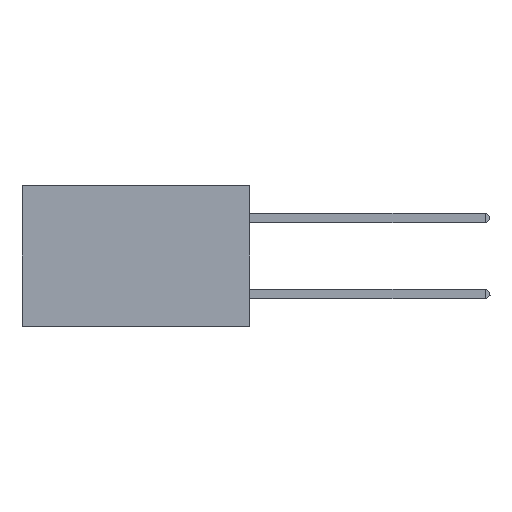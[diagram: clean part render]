
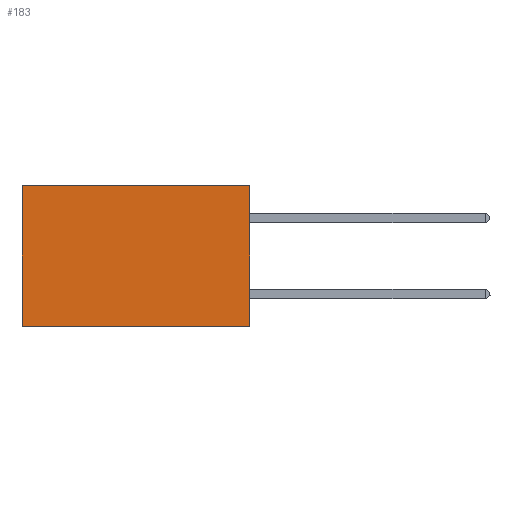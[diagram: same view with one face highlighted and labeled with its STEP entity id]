
A CAD part, left-side view. The second image highlights one B-rep face of the part: STEP entity #183.
In plain terms, the highlighted planar face has unit normal (-1, 0, 0).
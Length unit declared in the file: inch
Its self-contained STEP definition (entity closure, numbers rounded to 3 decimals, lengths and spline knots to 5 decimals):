
#183 = ADVANCED_FACE ( 'NONE', ( #19137 ), #21344, .F. ) ;
#465 = LINE ( 'NONE', #4104, #26621 ) ;
#587 = VECTOR ( 'NONE', #28675, 39.37008 ) ;
#904 = VERTEX_POINT ( 'NONE', #18651 ) ;
#2694 = AXIS2_PLACEMENT_3D ( 'NONE', #28165, #21142, #10325 ) ;
#4104 = CARTESIAN_POINT ( 'NONE',  ( 0.2875, 0.6, 0. ) ) ;
#4763 = ORIENTED_EDGE ( 'NONE', *, *, #7177, .T. ) ;
#5711 = DIRECTION ( 'NONE',  ( 0., 0., -1. ) ) ;
#6086 = VECTOR ( 'NONE', #22652, 39.37008 ) ;
#6959 = VECTOR ( 'NONE', #5711, 39.37008 ) ;
#7177 = EDGE_CURVE ( 'NONE', #10884, #16559, #465, .T. ) ;
#7529 = LINE ( 'NONE', #8794, #587 ) ;
#7625 = CARTESIAN_POINT ( 'NONE',  ( 0.2875, 0.6, 0. ) ) ;
#7751 = DIRECTION ( 'NONE',  ( 0., 0., -1. ) ) ;
#8175 = CARTESIAN_POINT ( 'NONE',  ( 0.2875, 0.6, -0.37 ) ) ;
#8794 = CARTESIAN_POINT ( 'NONE',  ( 0.2875, 0., -0.37 ) ) ;
#9261 = EDGE_CURVE ( 'NONE', #904, #20827, #15377, .T. ) ;
#9324 = EDGE_LOOP ( 'NONE', ( #4763, #24900, #26496, #24456 ) ) ;
#9924 = CARTESIAN_POINT ( 'NONE',  ( 0.2875, 0., 0. ) ) ;
#10039 = CARTESIAN_POINT ( 'NONE',  ( 0.2875, 0., -0.37 ) ) ;
#10325 = DIRECTION ( 'NONE',  ( 0., 0., -1. ) ) ;
#10884 = VERTEX_POINT ( 'NONE', #7625 ) ;
#14539 = EDGE_CURVE ( 'NONE', #904, #10884, #24881, .T. ) ;
#15377 = LINE ( 'NONE', #27958, #6959 ) ;
#16559 = VERTEX_POINT ( 'NONE', #8175 ) ;
#18651 = CARTESIAN_POINT ( 'NONE',  ( 0.2875, 0., 0. ) ) ;
#19137 = FACE_OUTER_BOUND ( 'NONE', #9324, .T. ) ;
#20827 = VERTEX_POINT ( 'NONE', #10039 ) ;
#21142 = DIRECTION ( 'NONE',  ( 1., 0., 0. ) ) ;
#21344 = PLANE ( 'NONE',  #2694 ) ;
#22652 = DIRECTION ( 'NONE',  ( 0., 1., 0. ) ) ;
#24456 = ORIENTED_EDGE ( 'NONE', *, *, #14539, .T. ) ;
#24881 = LINE ( 'NONE', #9924, #6086 ) ;
#24900 = ORIENTED_EDGE ( 'NONE', *, *, #27863, .F. ) ;
#26496 = ORIENTED_EDGE ( 'NONE', *, *, #9261, .F. ) ;
#26621 = VECTOR ( 'NONE', #7751, 39.37008 ) ;
#27863 = EDGE_CURVE ( 'NONE', #20827, #16559, #7529, .T. ) ;
#27958 = CARTESIAN_POINT ( 'NONE',  ( 0.2875, 0., 0. ) ) ;
#28165 = CARTESIAN_POINT ( 'NONE',  ( 0.2875, 0., 0. ) ) ;
#28675 = DIRECTION ( 'NONE',  ( 0., 1., 0. ) ) ;
